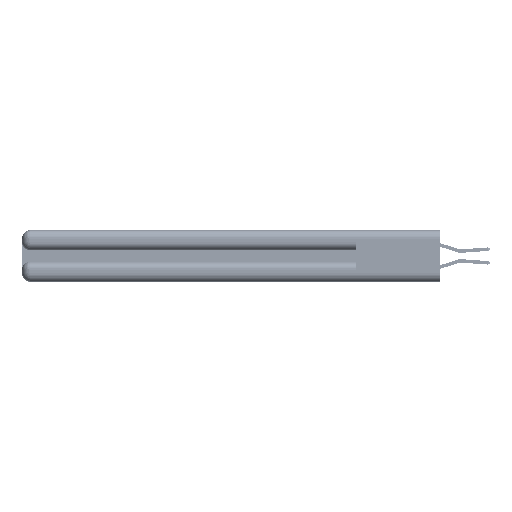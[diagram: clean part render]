
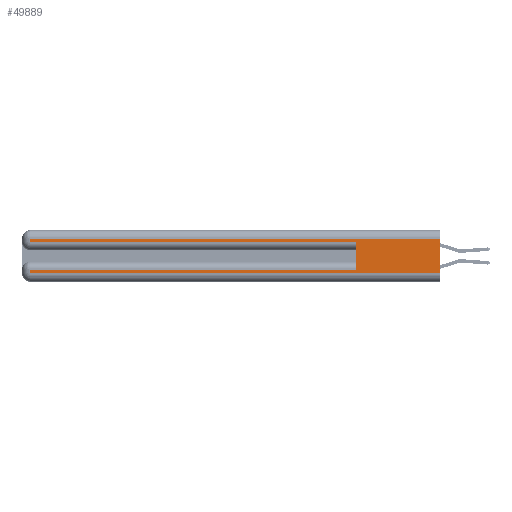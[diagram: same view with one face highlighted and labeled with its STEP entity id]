
A CAD part, left-side view. The second image highlights one B-rep face of the part: STEP entity #49889.
In plain terms, the highlighted planar face has unit normal (-1, 0, 0).
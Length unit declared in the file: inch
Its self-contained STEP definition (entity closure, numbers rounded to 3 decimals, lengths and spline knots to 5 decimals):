
#427 = EDGE_CURVE ( 'NONE', #15119, #26285, #36112, .T. ) ;
#1332 = VECTOR ( 'NONE', #12035, 39.37008 ) ;
#1731 = EDGE_CURVE ( 'NONE', #27163, #24331, #26500, .T. ) ;
#6256 = EDGE_CURVE ( 'NONE', #26145, #15119, #39851, .T. ) ;
#6346 = ORIENTED_EDGE ( 'NONE', *, *, #427, .T. ) ;
#7165 = CARTESIAN_POINT ( 'NONE',  ( 0., 0.6, 0.285 ) ) ;
#7812 = ORIENTED_EDGE ( 'NONE', *, *, #34723, .F. ) ;
#10381 = VECTOR ( 'NONE', #36711, 39.37008 ) ;
#12035 = DIRECTION ( 'NONE',  ( 0., -1., 0. ) ) ;
#13243 = ORIENTED_EDGE ( 'NONE', *, *, #20421, .T. ) ;
#13272 = ORIENTED_EDGE ( 'NONE', *, *, #6256, .T. ) ;
#13559 = DIRECTION ( 'NONE',  ( 1., 0., 0. ) ) ;
#14984 = CARTESIAN_POINT ( 'NONE',  ( 0., 0.6, 0.145 ) ) ;
#15119 = VERTEX_POINT ( 'NONE', #16847 ) ;
#15493 = VERTEX_POINT ( 'NONE', #41009 ) ;
#15534 = EDGE_CURVE ( 'NONE', #40825, #26145, #40352, .T. ) ;
#15692 = CARTESIAN_POINT ( 'NONE',  ( 0., 2.94, 0.31 ) ) ;
#16847 = CARTESIAN_POINT ( 'NONE',  ( 0., 2.94, 0.285 ) ) ;
#17439 = ORIENTED_EDGE ( 'NONE', *, *, #15534, .T. ) ;
#18075 = ORIENTED_EDGE ( 'NONE', *, *, #36242, .F. ) ;
#20421 = EDGE_CURVE ( 'NONE', #24331, #15493, #34634, .T. ) ;
#21882 = FACE_OUTER_BOUND ( 'NONE', #55513, .T. ) ;
#22688 = AXIS2_PLACEMENT_3D ( 'NONE', #52811, #13559, #39279 ) ;
#23133 = CARTESIAN_POINT ( 'NONE',  ( 0., 0., 0.06 ) ) ;
#24331 = VERTEX_POINT ( 'NONE', #25827 ) ;
#24896 = CARTESIAN_POINT ( 'NONE',  ( 0., 2.94, 0.37 ) ) ;
#25113 = DIRECTION ( 'NONE',  ( 0., 0., -1. ) ) ;
#25827 = CARTESIAN_POINT ( 'NONE',  ( 0., 2.94, 0.085 ) ) ;
#26145 = VERTEX_POINT ( 'NONE', #15692 ) ;
#26159 = DIRECTION ( 'NONE',  ( 0., 0., -1. ) ) ;
#26274 = CARTESIAN_POINT ( 'NONE',  ( 0., 0.6, 0.085 ) ) ;
#26285 = VERTEX_POINT ( 'NONE', #7165 ) ;
#26500 = LINE ( 'NONE', #53989, #55786 ) ;
#27163 = VERTEX_POINT ( 'NONE', #26274 ) ;
#28231 = DIRECTION ( 'NONE',  ( 0., 1., 0. ) ) ;
#29564 = CARTESIAN_POINT ( 'NONE',  ( 0., 0., 0.06 ) ) ;
#30967 = VECTOR ( 'NONE', #26159, 39.37008 ) ;
#31904 = EDGE_CURVE ( 'NONE', #15493, #35272, #31958, .T. ) ;
#31958 = LINE ( 'NONE', #29564, #1332 ) ;
#34634 = LINE ( 'NONE', #24896, #53740 ) ;
#34723 = EDGE_CURVE ( 'NONE', #27163, #26285, #47897, .T. ) ;
#35272 = VERTEX_POINT ( 'NONE', #23133 ) ;
#36112 = LINE ( 'NONE', #49180, #47065 ) ;
#36242 = EDGE_CURVE ( 'NONE', #40825, #35272, #53371, .T. ) ;
#36711 = DIRECTION ( 'NONE',  ( 0., 0., 1. ) ) ;
#36758 = DIRECTION ( 'NONE',  ( 0., -1., 0. ) ) ;
#37548 = VECTOR ( 'NONE', #40642, 39.37008 ) ;
#37855 = DIRECTION ( 'NONE',  ( 0., 0., -1. ) ) ;
#39279 = DIRECTION ( 'NONE',  ( 0., 0., -1. ) ) ;
#39851 = LINE ( 'NONE', #48069, #30967 ) ;
#40352 = LINE ( 'NONE', #41197, #37548 ) ;
#40642 = DIRECTION ( 'NONE',  ( 0., 1., 0. ) ) ;
#40825 = VERTEX_POINT ( 'NONE', #54176 ) ;
#41009 = CARTESIAN_POINT ( 'NONE',  ( 0., 2.94, 0.06 ) ) ;
#41091 = ORIENTED_EDGE ( 'NONE', *, *, #1731, .T. ) ;
#41197 = CARTESIAN_POINT ( 'NONE',  ( 0., 0., 0.31 ) ) ;
#41753 = VECTOR ( 'NONE', #25113, 39.37008 ) ;
#44053 = PLANE ( 'NONE',  #22688 ) ;
#47065 = VECTOR ( 'NONE', #36758, 39.37008 ) ;
#47806 = CARTESIAN_POINT ( 'NONE',  ( 0., 0., 0.37 ) ) ;
#47897 = LINE ( 'NONE', #14984, #10381 ) ;
#48069 = CARTESIAN_POINT ( 'NONE',  ( 0., 2.94, 0.37 ) ) ;
#49180 = CARTESIAN_POINT ( 'NONE',  ( 0., 0., 0.285 ) ) ;
#49889 = ADVANCED_FACE ( 'NONE', ( #21882 ), #44053, .F. ) ;
#50770 = ORIENTED_EDGE ( 'NONE', *, *, #31904, .T. ) ;
#52811 = CARTESIAN_POINT ( 'NONE',  ( 0., 0., 0.37 ) ) ;
#53371 = LINE ( 'NONE', #47806, #41753 ) ;
#53740 = VECTOR ( 'NONE', #37855, 39.37008 ) ;
#53989 = CARTESIAN_POINT ( 'NONE',  ( 0., 0., 0.085 ) ) ;
#54176 = CARTESIAN_POINT ( 'NONE',  ( 0., 0., 0.31 ) ) ;
#55513 = EDGE_LOOP ( 'NONE', ( #18075, #17439, #13272, #6346, #7812, #41091, #13243, #50770 ) ) ;
#55786 = VECTOR ( 'NONE', #28231, 39.37008 ) ;
